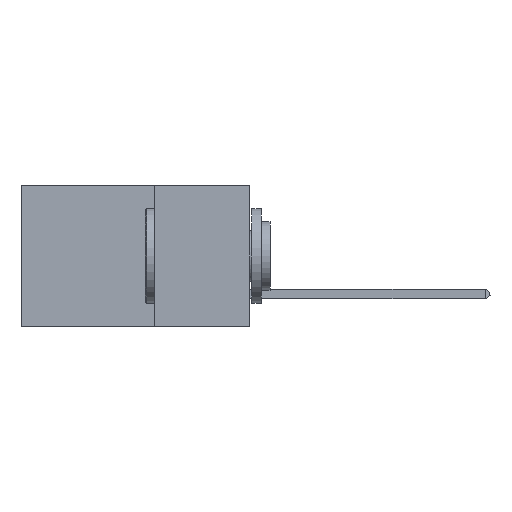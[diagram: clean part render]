
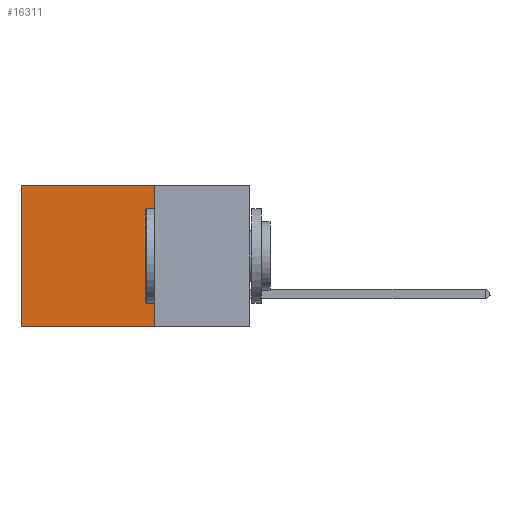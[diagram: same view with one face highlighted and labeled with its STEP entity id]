
A CAD part, left-side view. The second image highlights one B-rep face of the part: STEP entity #16311.
In plain terms, the highlighted planar face has unit normal (-1, 0, 0).
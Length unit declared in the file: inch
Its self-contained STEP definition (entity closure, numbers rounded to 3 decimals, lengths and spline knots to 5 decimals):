
#351 = VECTOR ( 'NONE', #12072, 39.37008 ) ;
#808 = PLANE ( 'NONE',  #25021 ) ;
#1128 = LINE ( 'NONE', #26965, #6563 ) ;
#1398 = CARTESIAN_POINT ( 'NONE',  ( 0.2875, 0.25, 0. ) ) ;
#1437 = CARTESIAN_POINT ( 'NONE',  ( 0.2875, 0.25, -0.37 ) ) ;
#1826 = ORIENTED_EDGE ( 'NONE', *, *, #23455, .T. ) ;
#2408 = CARTESIAN_POINT ( 'NONE',  ( 0.2875, 0.6, -0.37 ) ) ;
#2646 = LINE ( 'NONE', #14655, #22195 ) ;
#2910 = CARTESIAN_POINT ( 'NONE',  ( 0.2875, 0.25, 0. ) ) ;
#4032 = CARTESIAN_POINT ( 'NONE',  ( 0.2875, 0.6, 0. ) ) ;
#4420 = EDGE_CURVE ( 'NONE', #15398, #7658, #13199, .T. ) ;
#4671 = DIRECTION ( 'NONE',  ( 0., 0., -1. ) ) ;
#6068 = VECTOR ( 'NONE', #4671, 39.37008 ) ;
#6563 = VECTOR ( 'NONE', #26870, 39.37008 ) ;
#6991 = VERTEX_POINT ( 'NONE', #20750 ) ;
#7242 = DIRECTION ( 'NONE',  ( 0., 0., -1. ) ) ;
#7658 = VERTEX_POINT ( 'NONE', #2408 ) ;
#8038 = VERTEX_POINT ( 'NONE', #1437 ) ;
#10339 = FACE_OUTER_BOUND ( 'NONE', #19507, .T. ) ;
#12072 = DIRECTION ( 'NONE',  ( 0., 0., -1. ) ) ;
#13199 = LINE ( 'NONE', #4032, #6068 ) ;
#14093 = ORIENTED_EDGE ( 'NONE', *, *, #22129, .F. ) ;
#14655 = CARTESIAN_POINT ( 'NONE',  ( 0.2875, 0.25, 0. ) ) ;
#14917 = CARTESIAN_POINT ( 'NONE',  ( 0.2875, 0.6, 0. ) ) ;
#15398 = VERTEX_POINT ( 'NONE', #14917 ) ;
#16311 = ADVANCED_FACE ( 'NONE', ( #10339 ), #808, .F. ) ;
#17403 = EDGE_CURVE ( 'NONE', #8038, #7658, #1128, .T. ) ;
#18067 = ORIENTED_EDGE ( 'NONE', *, *, #17403, .F. ) ;
#18280 = LINE ( 'NONE', #1398, #351 ) ;
#18673 = ORIENTED_EDGE ( 'NONE', *, *, #4420, .T. ) ;
#19507 = EDGE_LOOP ( 'NONE', ( #18673, #18067, #14093, #1826 ) ) ;
#20382 = DIRECTION ( 'NONE',  ( 1., 0., 0. ) ) ;
#20750 = CARTESIAN_POINT ( 'NONE',  ( 0.2875, 0.25, 0. ) ) ;
#22129 = EDGE_CURVE ( 'NONE', #6991, #8038, #18280, .T. ) ;
#22195 = VECTOR ( 'NONE', #25116, 39.37008 ) ;
#23455 = EDGE_CURVE ( 'NONE', #6991, #15398, #2646, .T. ) ;
#25021 = AXIS2_PLACEMENT_3D ( 'NONE', #2910, #20382, #7242 ) ;
#25116 = DIRECTION ( 'NONE',  ( 0., 1., 0. ) ) ;
#26870 = DIRECTION ( 'NONE',  ( 0., 1., 0. ) ) ;
#26965 = CARTESIAN_POINT ( 'NONE',  ( 0.2875, 0.25, -0.37 ) ) ;
